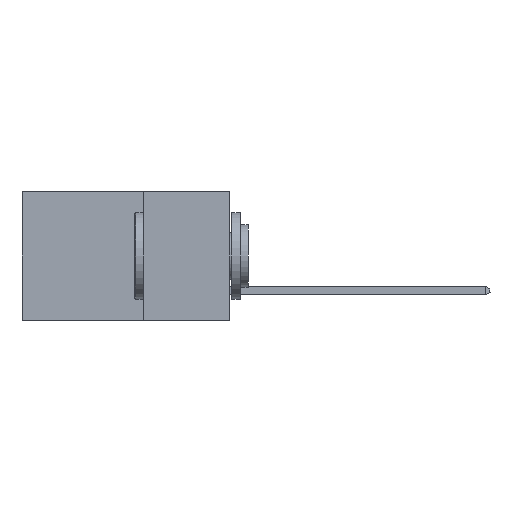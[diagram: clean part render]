
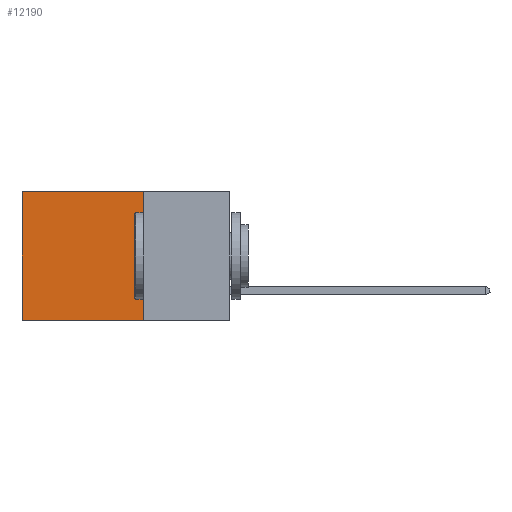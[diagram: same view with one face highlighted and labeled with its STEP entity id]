
A CAD part, left-side view. The second image highlights one B-rep face of the part: STEP entity #12190.
In plain terms, the highlighted planar face has unit normal (-1, 0, 0).
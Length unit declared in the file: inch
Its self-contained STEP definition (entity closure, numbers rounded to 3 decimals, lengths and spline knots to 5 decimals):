
#354 = VERTEX_POINT ( 'NONE', #3627 ) ;
#723 = CARTESIAN_POINT ( 'NONE',  ( 0.298, 0.6, 0. ) ) ;
#1489 = CARTESIAN_POINT ( 'NONE',  ( 0.298, 0.25, 0. ) ) ;
#1954 = LINE ( 'NONE', #16325, #17912 ) ;
#3627 = CARTESIAN_POINT ( 'NONE',  ( 0.298, 0.25, -0.37 ) ) ;
#5905 = LINE ( 'NONE', #8237, #6613 ) ;
#5944 = PLANE ( 'NONE',  #6537 ) ;
#6003 = FACE_OUTER_BOUND ( 'NONE', #18929, .T. ) ;
#6133 = EDGE_CURVE ( 'NONE', #25140, #7616, #6423, .T. ) ;
#6423 = LINE ( 'NONE', #9412, #26825 ) ;
#6537 = AXIS2_PLACEMENT_3D ( 'NONE', #1489, #8058, #20947 ) ;
#6613 = VECTOR ( 'NONE', #8037, 39.37008 ) ;
#7616 = VERTEX_POINT ( 'NONE', #21110 ) ;
#8037 = DIRECTION ( 'NONE',  ( 0., 1., 0. ) ) ;
#8058 = DIRECTION ( 'NONE',  ( 1., 0., 0. ) ) ;
#8237 = CARTESIAN_POINT ( 'NONE',  ( 0.298, 0.25, -0.37 ) ) ;
#9412 = CARTESIAN_POINT ( 'NONE',  ( 0.298, 0.25, 0. ) ) ;
#9492 = DIRECTION ( 'NONE',  ( 0., 0., -1. ) ) ;
#9620 = ORIENTED_EDGE ( 'NONE', *, *, #11951, .F. ) ;
#11923 = ORIENTED_EDGE ( 'NONE', *, *, #19418, .F. ) ;
#11951 = EDGE_CURVE ( 'NONE', #25140, #354, #1954, .T. ) ;
#12190 = ADVANCED_FACE ( 'NONE', ( #6003 ), #5944, .F. ) ;
#12285 = CARTESIAN_POINT ( 'NONE',  ( 0.298, 0.25, 0. ) ) ;
#13009 = VECTOR ( 'NONE', #9492, 39.37008 ) ;
#15258 = EDGE_CURVE ( 'NONE', #7616, #18992, #27641, .T. ) ;
#15526 = ORIENTED_EDGE ( 'NONE', *, *, #6133, .T. ) ;
#16325 = CARTESIAN_POINT ( 'NONE',  ( 0.298, 0.25, 0. ) ) ;
#17912 = VECTOR ( 'NONE', #22889, 39.37008 ) ;
#18929 = EDGE_LOOP ( 'NONE', ( #22132, #11923, #9620, #15526 ) ) ;
#18992 = VERTEX_POINT ( 'NONE', #22022 ) ;
#19418 = EDGE_CURVE ( 'NONE', #354, #18992, #5905, .T. ) ;
#20304 = DIRECTION ( 'NONE',  ( 0., 1., 0. ) ) ;
#20947 = DIRECTION ( 'NONE',  ( 0., 0., -1. ) ) ;
#21110 = CARTESIAN_POINT ( 'NONE',  ( 0.298, 0.6, 0. ) ) ;
#22022 = CARTESIAN_POINT ( 'NONE',  ( 0.298, 0.6, -0.37 ) ) ;
#22132 = ORIENTED_EDGE ( 'NONE', *, *, #15258, .T. ) ;
#22889 = DIRECTION ( 'NONE',  ( 0., 0., -1. ) ) ;
#25140 = VERTEX_POINT ( 'NONE', #12285 ) ;
#26825 = VECTOR ( 'NONE', #20304, 39.37008 ) ;
#27641 = LINE ( 'NONE', #723, #13009 ) ;
